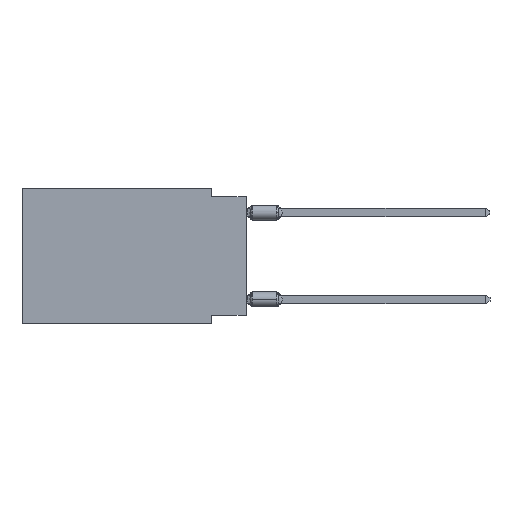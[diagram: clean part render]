
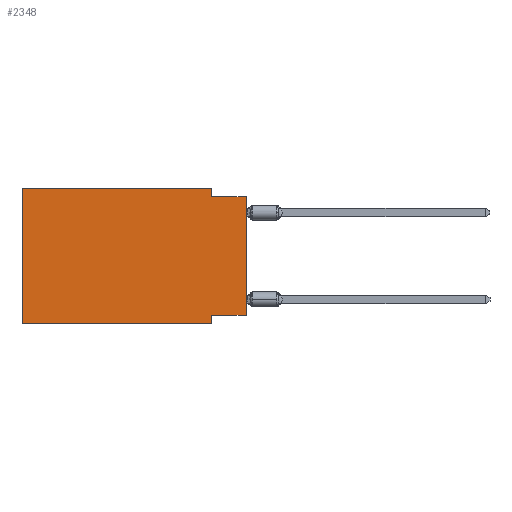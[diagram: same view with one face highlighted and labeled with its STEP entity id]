
A CAD part, left-side view. The second image highlights one B-rep face of the part: STEP entity #2348.
In plain terms, the highlighted planar face has unit normal (-1, 0, 0).
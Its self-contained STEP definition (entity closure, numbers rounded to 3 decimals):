
#337 = DIRECTION ( 'NONE',  ( 1., 0., 0. ) ) ;
#993 = EDGE_CURVE ( 'NONE', #15740, #12909, #19115, .T. ) ;
#1171 = VECTOR ( 'NONE', #17919, 1000. ) ;
#1552 = CARTESIAN_POINT ( 'NONE',  ( 0., 2.54, -0.635 ) ) ;
#1657 = VECTOR ( 'NONE', #8726, 1000. ) ;
#2113 = VERTEX_POINT ( 'NONE', #12676 ) ;
#2348 = ADVANCED_FACE ( 'NONE', ( #23247 ), #16139, .F. ) ;
#2833 = VERTEX_POINT ( 'NONE', #18180 ) ;
#3126 = DIRECTION ( 'NONE',  ( 0., -1., 0. ) ) ;
#4287 = EDGE_CURVE ( 'NONE', #14697, #7071, #19660, .T. ) ;
#4336 = VERTEX_POINT ( 'NONE', #1552 ) ;
#4356 = CARTESIAN_POINT ( 'NONE',  ( 0., 16.383, 0. ) ) ;
#5210 = EDGE_CURVE ( 'NONE', #9850, #4336, #8080, .T. ) ;
#5349 = CARTESIAN_POINT ( 'NONE',  ( 0., 0., 0. ) ) ;
#7071 = VERTEX_POINT ( 'NONE', #23414 ) ;
#7155 = VECTOR ( 'NONE', #14532, 1000. ) ;
#7349 = ORIENTED_EDGE ( 'NONE', *, *, #12714, .F. ) ;
#7456 = CARTESIAN_POINT ( 'NONE',  ( 0., 16.383, 0. ) ) ;
#7473 = CARTESIAN_POINT ( 'NONE',  ( 0., 2.54, -9.271 ) ) ;
#8080 = LINE ( 'NONE', #10030, #1171 ) ;
#8092 = EDGE_CURVE ( 'NONE', #15740, #7071, #18548, .T. ) ;
#8098 = EDGE_CURVE ( 'NONE', #2113, #14697, #24731, .T. ) ;
#8726 = DIRECTION ( 'NONE',  ( 0., 0., 1. ) ) ;
#8925 = ORIENTED_EDGE ( 'NONE', *, *, #5210, .F. ) ;
#9409 = AXIS2_PLACEMENT_3D ( 'NONE', #4356, #337, #9801 ) ;
#9801 = DIRECTION ( 'NONE',  ( 0., 0., -1. ) ) ;
#9850 = VERTEX_POINT ( 'NONE', #16115 ) ;
#9869 = ORIENTED_EDGE ( 'NONE', *, *, #8098, .F. ) ;
#9968 = CARTESIAN_POINT ( 'NONE',  ( 0., 2.54, -9.906 ) ) ;
#10030 = CARTESIAN_POINT ( 'NONE',  ( 0., 2.54, 0. ) ) ;
#10076 = ORIENTED_EDGE ( 'NONE', *, *, #993, .F. ) ;
#10492 = EDGE_LOOP ( 'NONE', ( #17064, #7349, #8925, #10820, #10076, #17149, #13546, #9869 ) ) ;
#10820 = ORIENTED_EDGE ( 'NONE', *, *, #22697, .F. ) ;
#12676 = CARTESIAN_POINT ( 'NONE',  ( 0., 0., -9.271 ) ) ;
#12714 = EDGE_CURVE ( 'NONE', #4336, #2833, #21111, .T. ) ;
#12909 = VERTEX_POINT ( 'NONE', #14245 ) ;
#13030 = CARTESIAN_POINT ( 'NONE',  ( 0., 16.383, -9.906 ) ) ;
#13546 = ORIENTED_EDGE ( 'NONE', *, *, #4287, .F. ) ;
#13606 = CARTESIAN_POINT ( 'NONE',  ( 0., 0., -0.635 ) ) ;
#14245 = CARTESIAN_POINT ( 'NONE',  ( 0., 16.383, 0. ) ) ;
#14532 = DIRECTION ( 'NONE',  ( 0., -1., 0. ) ) ;
#14697 = VERTEX_POINT ( 'NONE', #7473 ) ;
#14999 = EDGE_CURVE ( 'NONE', #2113, #2833, #18806, .T. ) ;
#15033 = DIRECTION ( 'NONE',  ( 0., 1., 0. ) ) ;
#15740 = VERTEX_POINT ( 'NONE', #13030 ) ;
#16115 = CARTESIAN_POINT ( 'NONE',  ( 0., 2.54, 0. ) ) ;
#16139 = PLANE ( 'NONE',  #9409 ) ;
#16613 = CARTESIAN_POINT ( 'NONE',  ( 0., 0., -9.271 ) ) ;
#16905 = VECTOR ( 'NONE', #23220, 1000. ) ;
#17064 = ORIENTED_EDGE ( 'NONE', *, *, #14999, .T. ) ;
#17149 = ORIENTED_EDGE ( 'NONE', *, *, #8092, .T. ) ;
#17287 = VECTOR ( 'NONE', #3126, 1000. ) ;
#17734 = DIRECTION ( 'NONE',  ( 0., 0., -1. ) ) ;
#17919 = DIRECTION ( 'NONE',  ( 0., 0., -1. ) ) ;
#18180 = CARTESIAN_POINT ( 'NONE',  ( 0., 0., -0.635 ) ) ;
#18548 = LINE ( 'NONE', #20357, #7155 ) ;
#18806 = LINE ( 'NONE', #5349, #1657 ) ;
#18989 = DIRECTION ( 'NONE',  ( 0., 0., 1. ) ) ;
#19115 = LINE ( 'NONE', #25318, #24809 ) ;
#19660 = LINE ( 'NONE', #9968, #24337 ) ;
#20357 = CARTESIAN_POINT ( 'NONE',  ( 0., 16.383, -9.906 ) ) ;
#21111 = LINE ( 'NONE', #13606, #17287 ) ;
#21542 = LINE ( 'NONE', #7456, #16905 ) ;
#22431 = VECTOR ( 'NONE', #15033, 1000. ) ;
#22697 = EDGE_CURVE ( 'NONE', #12909, #9850, #21542, .T. ) ;
#23220 = DIRECTION ( 'NONE',  ( 0., -1., 0. ) ) ;
#23247 = FACE_OUTER_BOUND ( 'NONE', #10492, .T. ) ;
#23414 = CARTESIAN_POINT ( 'NONE',  ( 0., 2.54, -9.906 ) ) ;
#24337 = VECTOR ( 'NONE', #17734, 1000. ) ;
#24731 = LINE ( 'NONE', #16613, #22431 ) ;
#24809 = VECTOR ( 'NONE', #18989, 1000. ) ;
#25318 = CARTESIAN_POINT ( 'NONE',  ( 0., 16.383, 0. ) ) ;
